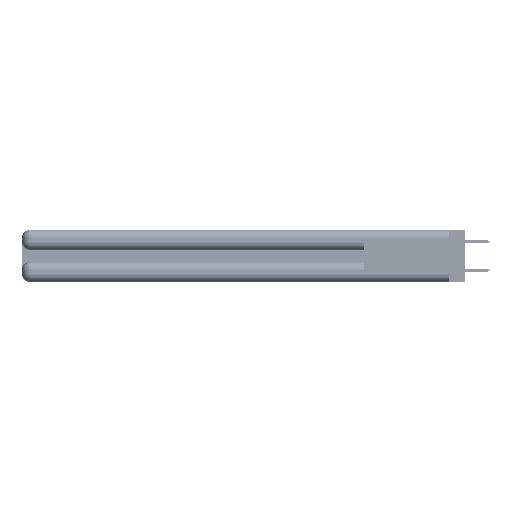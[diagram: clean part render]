
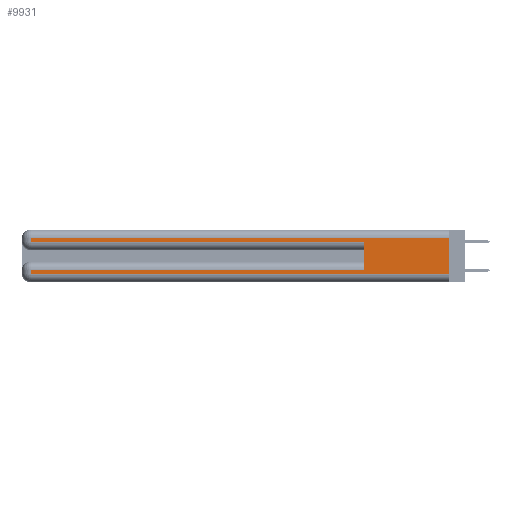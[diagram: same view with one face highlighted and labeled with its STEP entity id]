
A CAD part, left-side view. The second image highlights one B-rep face of the part: STEP entity #9931.
In plain terms, the highlighted planar face has unit normal (-1, 0, 0).
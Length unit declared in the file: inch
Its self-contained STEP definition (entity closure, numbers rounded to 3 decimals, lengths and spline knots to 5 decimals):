
#1417 = CARTESIAN_POINT ( 'NONE',  ( 0., 0.6, 0.285 ) ) ;
#3250 = ORIENTED_EDGE ( 'NONE', *, *, #57520, .F. ) ;
#3325 = LINE ( 'NONE', #22429, #12427 ) ;
#4325 = CARTESIAN_POINT ( 'NONE',  ( 0., 0., 0.06 ) ) ;
#5806 = EDGE_CURVE ( 'NONE', #8436, #7881, #28512, .T. ) ;
#7321 = LINE ( 'NONE', #7328, #53445 ) ;
#7328 = CARTESIAN_POINT ( 'NONE',  ( 0., 0.6, 0.145 ) ) ;
#7881 = VERTEX_POINT ( 'NONE', #32617 ) ;
#7940 = CARTESIAN_POINT ( 'NONE',  ( 0., 2.94, 0.31 ) ) ;
#8436 = VERTEX_POINT ( 'NONE', #54061 ) ;
#8464 = ORIENTED_EDGE ( 'NONE', *, *, #14263, .T. ) ;
#9213 = VERTEX_POINT ( 'NONE', #16792 ) ;
#9389 = EDGE_CURVE ( 'NONE', #35099, #35561, #3325, .T. ) ;
#9575 = FACE_OUTER_BOUND ( 'NONE', #47800, .T. ) ;
#9931 = ADVANCED_FACE ( 'NONE', ( #9575 ), #43801, .F. ) ;
#10058 = DIRECTION ( 'NONE',  ( 0., 0., -1. ) ) ;
#12138 = EDGE_CURVE ( 'NONE', #46917, #13938, #24357, .T. ) ;
#12427 = VECTOR ( 'NONE', #31393, 39.37008 ) ;
#12472 = VECTOR ( 'NONE', #53082, 39.37008 ) ;
#12692 = LINE ( 'NONE', #19185, #57463 ) ;
#13938 = VERTEX_POINT ( 'NONE', #7940 ) ;
#14263 = EDGE_CURVE ( 'NONE', #13938, #35099, #44307, .T. ) ;
#14372 = LINE ( 'NONE', #50756, #48558 ) ;
#15347 = VERTEX_POINT ( 'NONE', #41478 ) ;
#16660 = VECTOR ( 'NONE', #17292, 39.37008 ) ;
#16792 = CARTESIAN_POINT ( 'NONE',  ( 0., 2.94, 0.085 ) ) ;
#17094 = DIRECTION ( 'NONE',  ( 1., 0., 0. ) ) ;
#17292 = DIRECTION ( 'NONE',  ( 0., 0., -1. ) ) ;
#17348 = CARTESIAN_POINT ( 'NONE',  ( 0., 0., 0.31 ) ) ;
#18394 = EDGE_CURVE ( 'NONE', #9213, #8436, #50886, .T. ) ;
#19185 = CARTESIAN_POINT ( 'NONE',  ( 0., 0., 0.37 ) ) ;
#19723 = CARTESIAN_POINT ( 'NONE',  ( 0., 0., 0.31 ) ) ;
#22429 = CARTESIAN_POINT ( 'NONE',  ( 0., 0., 0.285 ) ) ;
#23993 = DIRECTION ( 'NONE',  ( 0., 1., 0. ) ) ;
#24357 = LINE ( 'NONE', #17348, #12472 ) ;
#24494 = ORIENTED_EDGE ( 'NONE', *, *, #12138, .T. ) ;
#25346 = ORIENTED_EDGE ( 'NONE', *, *, #18394, .T. ) ;
#27821 = CARTESIAN_POINT ( 'NONE',  ( 0., 2.94, 0.37 ) ) ;
#28512 = LINE ( 'NONE', #4325, #40391 ) ;
#29446 = ORIENTED_EDGE ( 'NONE', *, *, #35065, .F. ) ;
#31054 = VECTOR ( 'NONE', #10058, 39.37008 ) ;
#31393 = DIRECTION ( 'NONE',  ( 0., -1., 0. ) ) ;
#32617 = CARTESIAN_POINT ( 'NONE',  ( 0., 0., 0.06 ) ) ;
#35065 = EDGE_CURVE ( 'NONE', #15347, #35561, #7321, .T. ) ;
#35099 = VERTEX_POINT ( 'NONE', #47514 ) ;
#35561 = VERTEX_POINT ( 'NONE', #1417 ) ;
#35585 = DIRECTION ( 'NONE',  ( 0., -1., 0. ) ) ;
#36926 = DIRECTION ( 'NONE',  ( 0., 0., -1. ) ) ;
#38586 = DIRECTION ( 'NONE',  ( 0., 0., 1. ) ) ;
#40391 = VECTOR ( 'NONE', #35585, 39.37008 ) ;
#41478 = CARTESIAN_POINT ( 'NONE',  ( 0., 0.6, 0.085 ) ) ;
#43801 = PLANE ( 'NONE',  #50641 ) ;
#44307 = LINE ( 'NONE', #27821, #31054 ) ;
#44837 = ORIENTED_EDGE ( 'NONE', *, *, #9389, .T. ) ;
#46903 = EDGE_CURVE ( 'NONE', #15347, #9213, #14372, .T. ) ;
#46917 = VERTEX_POINT ( 'NONE', #19723 ) ;
#47514 = CARTESIAN_POINT ( 'NONE',  ( 0., 2.94, 0.285 ) ) ;
#47800 = EDGE_LOOP ( 'NONE', ( #3250, #24494, #8464, #44837, #29446, #49024, #25346, #55478 ) ) ;
#48082 = CARTESIAN_POINT ( 'NONE',  ( 0., 0., 0.37 ) ) ;
#48279 = DIRECTION ( 'NONE',  ( 0., 0., -1. ) ) ;
#48446 = CARTESIAN_POINT ( 'NONE',  ( 0., 2.94, 0.37 ) ) ;
#48558 = VECTOR ( 'NONE', #23993, 39.37008 ) ;
#49024 = ORIENTED_EDGE ( 'NONE', *, *, #46903, .T. ) ;
#50641 = AXIS2_PLACEMENT_3D ( 'NONE', #48082, #17094, #48279 ) ;
#50756 = CARTESIAN_POINT ( 'NONE',  ( 0., 0., 0.085 ) ) ;
#50886 = LINE ( 'NONE', #48446, #16660 ) ;
#53082 = DIRECTION ( 'NONE',  ( 0., 1., 0. ) ) ;
#53445 = VECTOR ( 'NONE', #38586, 39.37008 ) ;
#54061 = CARTESIAN_POINT ( 'NONE',  ( 0., 2.94, 0.06 ) ) ;
#55478 = ORIENTED_EDGE ( 'NONE', *, *, #5806, .T. ) ;
#57463 = VECTOR ( 'NONE', #36926, 39.37008 ) ;
#57520 = EDGE_CURVE ( 'NONE', #46917, #7881, #12692, .T. ) ;
